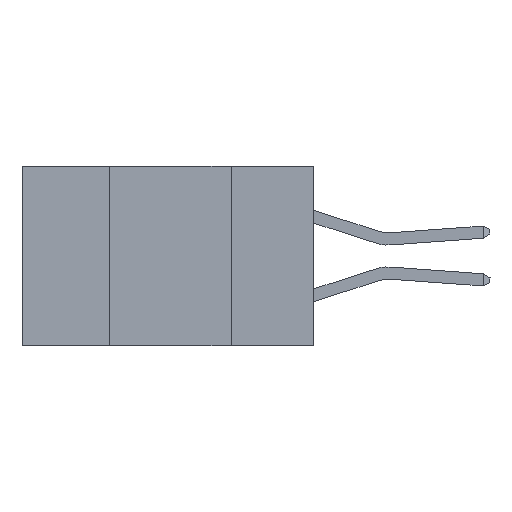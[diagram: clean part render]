
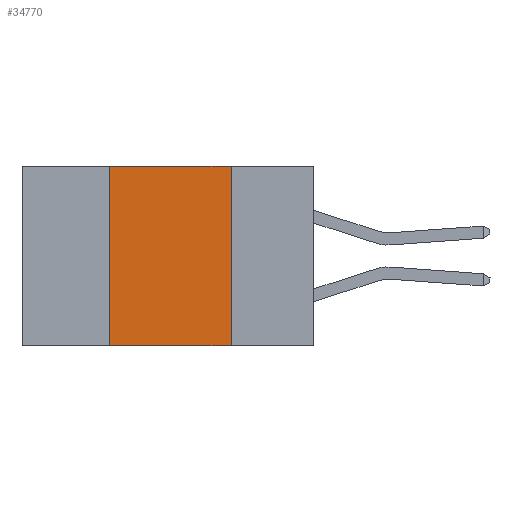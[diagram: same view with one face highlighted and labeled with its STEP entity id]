
A CAD part, left-side view. The second image highlights one B-rep face of the part: STEP entity #34770.
In plain terms, the highlighted planar face has unit normal (-1, 0, 0).
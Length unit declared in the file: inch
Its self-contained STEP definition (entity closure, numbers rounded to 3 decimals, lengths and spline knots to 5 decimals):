
#1684 = EDGE_LOOP ( 'NONE', ( #22326, #21137, #5209, #33434 ) ) ;
#3162 = VECTOR ( 'NONE', #38720, 39.37008 ) ;
#3377 = CARTESIAN_POINT ( 'NONE',  ( 0., 0.42, -0.37 ) ) ;
#3600 = CARTESIAN_POINT ( 'NONE',  ( 0., 0.17, -0.37 ) ) ;
#3755 = LINE ( 'NONE', #16151, #16729 ) ;
#4990 = EDGE_CURVE ( 'NONE', #12359, #5573, #3755, .T. ) ;
#5209 = ORIENTED_EDGE ( 'NONE', *, *, #4990, .F. ) ;
#5573 = VERTEX_POINT ( 'NONE', #27145 ) ;
#10656 = CARTESIAN_POINT ( 'NONE',  ( 0., 0.6, -0.37 ) ) ;
#11348 = LINE ( 'NONE', #30317, #26811 ) ;
#11545 = DIRECTION ( 'NONE',  ( 0., 0., -1. ) ) ;
#12025 = DIRECTION ( 'NONE',  ( 1., 0., 0. ) ) ;
#12359 = VERTEX_POINT ( 'NONE', #3377 ) ;
#13308 = CARTESIAN_POINT ( 'NONE',  ( 0., 0.6, 0. ) ) ;
#14040 = EDGE_CURVE ( 'NONE', #12359, #39891, #20560, .T. ) ;
#15639 = EDGE_CURVE ( 'NONE', #5573, #24067, #28568, .T. ) ;
#16151 = CARTESIAN_POINT ( 'NONE',  ( 0., 0.42, 0. ) ) ;
#16729 = VECTOR ( 'NONE', #28717, 39.37008 ) ;
#18216 = FACE_OUTER_BOUND ( 'NONE', #1684, .T. ) ;
#18298 = CARTESIAN_POINT ( 'NONE',  ( 0., 0.17, 0. ) ) ;
#20560 = LINE ( 'NONE', #10656, #3162 ) ;
#21137 = ORIENTED_EDGE ( 'NONE', *, *, #15639, .F. ) ;
#21588 = AXIS2_PLACEMENT_3D ( 'NONE', #21923, #12025, #24388 ) ;
#21923 = CARTESIAN_POINT ( 'NONE',  ( 0., 0.6, 0. ) ) ;
#22326 = ORIENTED_EDGE ( 'NONE', *, *, #33901, .F. ) ;
#24067 = VERTEX_POINT ( 'NONE', #18298 ) ;
#24388 = DIRECTION ( 'NONE',  ( 0., 0., -1. ) ) ;
#26811 = VECTOR ( 'NONE', #11545, 39.37008 ) ;
#27145 = CARTESIAN_POINT ( 'NONE',  ( 0., 0.42, 0. ) ) ;
#28568 = LINE ( 'NONE', #13308, #36217 ) ;
#28717 = DIRECTION ( 'NONE',  ( 0., 0., 1. ) ) ;
#30317 = CARTESIAN_POINT ( 'NONE',  ( 0., 0.17, 0. ) ) ;
#33434 = ORIENTED_EDGE ( 'NONE', *, *, #14040, .T. ) ;
#33901 = EDGE_CURVE ( 'NONE', #24067, #39891, #11348, .T. ) ;
#34770 = ADVANCED_FACE ( 'NONE', ( #18216 ), #40699, .F. ) ;
#34974 = DIRECTION ( 'NONE',  ( 0., -1., 0. ) ) ;
#36217 = VECTOR ( 'NONE', #34974, 39.37008 ) ;
#38720 = DIRECTION ( 'NONE',  ( 0., -1., 0. ) ) ;
#39891 = VERTEX_POINT ( 'NONE', #3600 ) ;
#40699 = PLANE ( 'NONE',  #21588 ) ;
